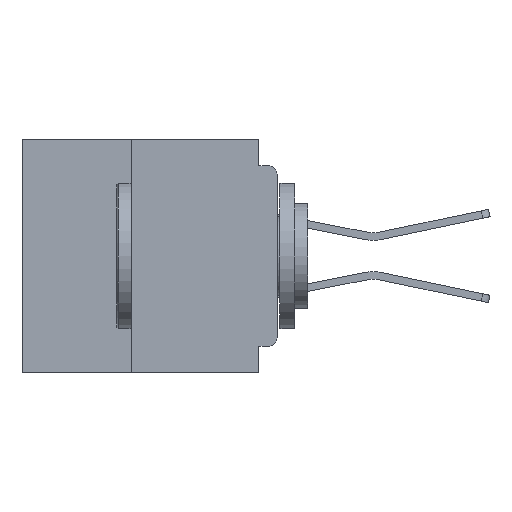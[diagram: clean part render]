
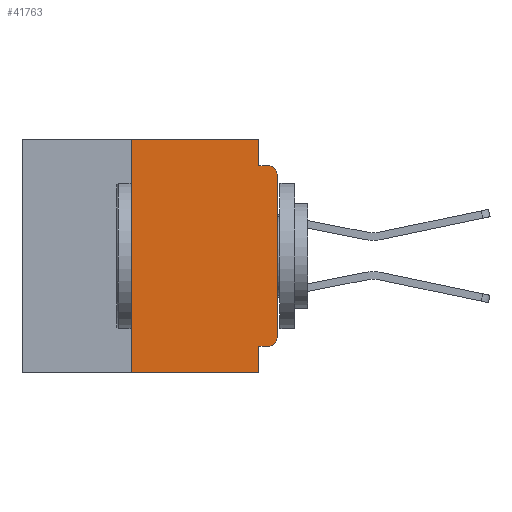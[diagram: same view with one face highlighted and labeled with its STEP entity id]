
A CAD part, left-side view. The second image highlights one B-rep face of the part: STEP entity #41763.
In plain terms, the highlighted planar face has unit normal (-1, 0, 0).
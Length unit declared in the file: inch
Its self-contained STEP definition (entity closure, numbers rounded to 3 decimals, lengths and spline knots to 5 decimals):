
#490 = EDGE_CURVE ( 'NONE', #9116, #26679, #37434, .T. ) ;
#535 = CARTESIAN_POINT ( 'NONE',  ( 0., 0.015, -0.045 ) ) ;
#658 = EDGE_CURVE ( 'NONE', #2965, #24181, #30311, .T. ) ;
#1085 = CARTESIAN_POINT ( 'NONE',  ( 0., 0.031, 0. ) ) ;
#2119 = EDGE_CURVE ( 'NONE', #2965, #22188, #32674, .T. ) ;
#2936 = CARTESIAN_POINT ( 'NONE',  ( 0., 0.25, -0.4 ) ) ;
#2965 = VERTEX_POINT ( 'NONE', #22588 ) ;
#2982 = CARTESIAN_POINT ( 'NONE',  ( 0., 0.25, 0. ) ) ;
#3753 = EDGE_CURVE ( 'NONE', #26679, #7637, #40191, .T. ) ;
#6242 = VECTOR ( 'NONE', #26413, 39.37008 ) ;
#6263 = CARTESIAN_POINT ( 'NONE',  ( 0., 0., 0. ) ) ;
#7279 = CARTESIAN_POINT ( 'NONE',  ( 0., 0., -0.06 ) ) ;
#7484 = ORIENTED_EDGE ( 'NONE', *, *, #17446, .F. ) ;
#7561 = VECTOR ( 'NONE', #31199, 39.37008 ) ;
#7637 = VERTEX_POINT ( 'NONE', #22737 ) ;
#7712 = CARTESIAN_POINT ( 'NONE',  ( 0., 0.25, -0.4 ) ) ;
#7886 = ORIENTED_EDGE ( 'NONE', *, *, #22337, .F. ) ;
#7997 = DIRECTION ( 'NONE',  ( -1., 0., 0. ) ) ;
#9116 = VERTEX_POINT ( 'NONE', #7712 ) ;
#9578 = VECTOR ( 'NONE', #40740, 39.37008 ) ;
#9633 = DIRECTION ( 'NONE',  ( 0., 0., 1. ) ) ;
#9942 = CARTESIAN_POINT ( 'NONE',  ( 0., 0., -0.34 ) ) ;
#10454 = VECTOR ( 'NONE', #11789, 39.37008 ) ;
#10982 = EDGE_CURVE ( 'NONE', #22188, #15398, #30261, .T. ) ;
#11048 = ORIENTED_EDGE ( 'NONE', *, *, #10982, .T. ) ;
#11522 = VECTOR ( 'NONE', #36458, 39.37008 ) ;
#11789 = DIRECTION ( 'NONE',  ( 0., -1., 0. ) ) ;
#12396 = CARTESIAN_POINT ( 'NONE',  ( 0., 0.031, -0.045 ) ) ;
#12931 = AXIS2_PLACEMENT_3D ( 'NONE', #29084, #35624, #16213 ) ;
#14860 = CARTESIAN_POINT ( 'NONE',  ( 0., 0.031, -0.4 ) ) ;
#15398 = VERTEX_POINT ( 'NONE', #7279 ) ;
#15724 = AXIS2_PLACEMENT_3D ( 'NONE', #27568, #7997, #30850 ) ;
#16213 = DIRECTION ( 'NONE',  ( 0., 0., -1. ) ) ;
#16522 = ORIENTED_EDGE ( 'NONE', *, *, #2119, .T. ) ;
#17089 = ORIENTED_EDGE ( 'NONE', *, *, #658, .F. ) ;
#17370 = EDGE_CURVE ( 'NONE', #15398, #25443, #37611, .T. ) ;
#17446 = EDGE_CURVE ( 'NONE', #24181, #27404, #19362, .T. ) ;
#18983 = EDGE_CURVE ( 'NONE', #7637, #37059, #27881, .T. ) ;
#19172 = LINE ( 'NONE', #34520, #10454 ) ;
#19362 = LINE ( 'NONE', #14860, #9578 ) ;
#19962 = CARTESIAN_POINT ( 'NONE',  ( 0., 0.031, -0.355 ) ) ;
#20249 = EDGE_CURVE ( 'NONE', #9116, #27404, #19172, .T. ) ;
#20549 = DIRECTION ( 'NONE',  ( 0., -1., 0. ) ) ;
#22188 = VERTEX_POINT ( 'NONE', #9942 ) ;
#22337 = EDGE_CURVE ( 'NONE', #37059, #25443, #39209, .T. ) ;
#22577 = PLANE ( 'NONE',  #12931 ) ;
#22588 = CARTESIAN_POINT ( 'NONE',  ( 0., 0.015, -0.355 ) ) ;
#22737 = CARTESIAN_POINT ( 'NONE',  ( 0., 0.031, 0. ) ) ;
#23176 = ORIENTED_EDGE ( 'NONE', *, *, #490, .F. ) ;
#24181 = VERTEX_POINT ( 'NONE', #19962 ) ;
#24288 = AXIS2_PLACEMENT_3D ( 'NONE', #39183, #38373, #38780 ) ;
#25443 = VERTEX_POINT ( 'NONE', #535 ) ;
#26137 = ORIENTED_EDGE ( 'NONE', *, *, #3753, .F. ) ;
#26413 = DIRECTION ( 'NONE',  ( 0., 1., 0. ) ) ;
#26679 = VERTEX_POINT ( 'NONE', #2982 ) ;
#26878 = VECTOR ( 'NONE', #33773, 39.37008 ) ;
#27404 = VERTEX_POINT ( 'NONE', #29722 ) ;
#27568 = CARTESIAN_POINT ( 'NONE',  ( 0., 0.015, -0.06 ) ) ;
#27881 = LINE ( 'NONE', #1085, #26878 ) ;
#27947 = ORIENTED_EDGE ( 'NONE', *, *, #20249, .T. ) ;
#29084 = CARTESIAN_POINT ( 'NONE',  ( 0., 0.437, 0. ) ) ;
#29722 = CARTESIAN_POINT ( 'NONE',  ( 0., 0.031, -0.4 ) ) ;
#30261 = LINE ( 'NONE', #6263, #39880 ) ;
#30311 = LINE ( 'NONE', #41413, #6242 ) ;
#30539 = EDGE_LOOP ( 'NONE', ( #11048, #40017, #7886, #34737, #26137, #23176, #27947, #7484, #17089, #16522 ) ) ;
#30633 = VECTOR ( 'NONE', #20549, 39.37008 ) ;
#30850 = DIRECTION ( 'NONE',  ( 0., 0., -1. ) ) ;
#31199 = DIRECTION ( 'NONE',  ( 0., -1., 0. ) ) ;
#31295 = CARTESIAN_POINT ( 'NONE',  ( 0., 0.437, 0. ) ) ;
#32674 = CIRCLE ( 'NONE', #24288, 0.015 ) ;
#33773 = DIRECTION ( 'NONE',  ( 0., 0., -1. ) ) ;
#34520 = CARTESIAN_POINT ( 'NONE',  ( 0., 0.437, -0.4 ) ) ;
#34737 = ORIENTED_EDGE ( 'NONE', *, *, #18983, .F. ) ;
#35624 = DIRECTION ( 'NONE',  ( 1., 0., 0. ) ) ;
#36458 = DIRECTION ( 'NONE',  ( 0., 0., 1. ) ) ;
#36714 = CARTESIAN_POINT ( 'NONE',  ( 0., 0., -0.045 ) ) ;
#37059 = VERTEX_POINT ( 'NONE', #12396 ) ;
#37434 = LINE ( 'NONE', #2936, #11522 ) ;
#37611 = CIRCLE ( 'NONE', #15724, 0.015 ) ;
#38373 = DIRECTION ( 'NONE',  ( -1., 0., 0. ) ) ;
#38780 = DIRECTION ( 'NONE',  ( 0., 0., -1. ) ) ;
#39183 = CARTESIAN_POINT ( 'NONE',  ( 0., 0.015, -0.34 ) ) ;
#39209 = LINE ( 'NONE', #36714, #30633 ) ;
#39880 = VECTOR ( 'NONE', #9633, 39.37008 ) ;
#40017 = ORIENTED_EDGE ( 'NONE', *, *, #17370, .T. ) ;
#40191 = LINE ( 'NONE', #31295, #7561 ) ;
#40740 = DIRECTION ( 'NONE',  ( 0., 0., -1. ) ) ;
#41413 = CARTESIAN_POINT ( 'NONE',  ( 0., 0., -0.355 ) ) ;
#41763 = ADVANCED_FACE ( 'NONE', ( #41980 ), #22577, .F. ) ;
#41980 = FACE_OUTER_BOUND ( 'NONE', #30539, .T. ) ;
